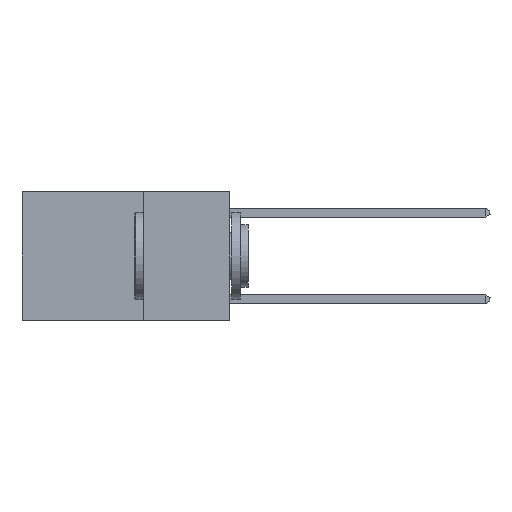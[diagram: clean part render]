
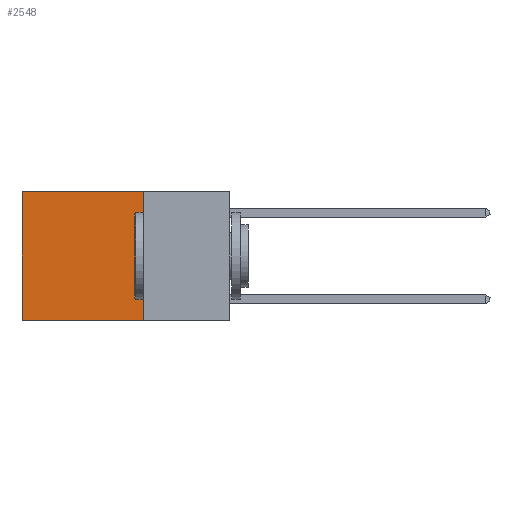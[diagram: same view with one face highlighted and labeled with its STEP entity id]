
A CAD part, left-side view. The second image highlights one B-rep face of the part: STEP entity #2548.
In plain terms, the highlighted planar face has unit normal (-1, 0, 0).
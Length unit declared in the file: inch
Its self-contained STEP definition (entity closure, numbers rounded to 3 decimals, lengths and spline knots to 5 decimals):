
#1246 = LINE ( 'NONE', #11704, #24470 ) ;
#1625 = FACE_OUTER_BOUND ( 'NONE', #7494, .T. ) ;
#2342 = CARTESIAN_POINT ( 'NONE',  ( 0.2625, 0.6, 0. ) ) ;
#2548 = ADVANCED_FACE ( 'NONE', ( #1625 ), #23971, .F. ) ;
#2975 = VERTEX_POINT ( 'NONE', #23609 ) ;
#3183 = VERTEX_POINT ( 'NONE', #4037 ) ;
#3497 = DIRECTION ( 'NONE',  ( 0., 0., -1. ) ) ;
#3573 = VECTOR ( 'NONE', #12818, 39.37008 ) ;
#4037 = CARTESIAN_POINT ( 'NONE',  ( 0.2625, 0.6, -0.37 ) ) ;
#5494 = CARTESIAN_POINT ( 'NONE',  ( 0.2625, 0.25, 0. ) ) ;
#5619 = CARTESIAN_POINT ( 'NONE',  ( 0.2625, 0.25, 0. ) ) ;
#5970 = EDGE_CURVE ( 'NONE', #22294, #3183, #23119, .T. ) ;
#7494 = EDGE_LOOP ( 'NONE', ( #20747, #15572, #9343, #20399 ) ) ;
#8528 = EDGE_CURVE ( 'NONE', #20217, #3183, #1246, .T. ) ;
#8768 = LINE ( 'NONE', #21359, #3573 ) ;
#8791 = VECTOR ( 'NONE', #21560, 39.37008 ) ;
#9343 = ORIENTED_EDGE ( 'NONE', *, *, #22044, .F. ) ;
#11704 = CARTESIAN_POINT ( 'NONE',  ( 0.2625, 0.6, 0. ) ) ;
#12243 = EDGE_CURVE ( 'NONE', #2975, #20217, #8768, .T. ) ;
#12818 = DIRECTION ( 'NONE',  ( 0., 1., 0. ) ) ;
#13393 = LINE ( 'NONE', #5619, #8791 ) ;
#15572 = ORIENTED_EDGE ( 'NONE', *, *, #5970, .F. ) ;
#17355 = CARTESIAN_POINT ( 'NONE',  ( 0.2625, 0.25, -0.37 ) ) ;
#19055 = AXIS2_PLACEMENT_3D ( 'NONE', #5494, #24105, #3497 ) ;
#19113 = DIRECTION ( 'NONE',  ( 0., 1., 0. ) ) ;
#19296 = CARTESIAN_POINT ( 'NONE',  ( 0.2625, 0.25, -0.37 ) ) ;
#20217 = VERTEX_POINT ( 'NONE', #2342 ) ;
#20399 = ORIENTED_EDGE ( 'NONE', *, *, #12243, .T. ) ;
#20747 = ORIENTED_EDGE ( 'NONE', *, *, #8528, .T. ) ;
#21359 = CARTESIAN_POINT ( 'NONE',  ( 0.2625, 0.25, 0. ) ) ;
#21560 = DIRECTION ( 'NONE',  ( 0., 0., -1. ) ) ;
#22044 = EDGE_CURVE ( 'NONE', #2975, #22294, #13393, .T. ) ;
#22294 = VERTEX_POINT ( 'NONE', #19296 ) ;
#23119 = LINE ( 'NONE', #17355, #25457 ) ;
#23609 = CARTESIAN_POINT ( 'NONE',  ( 0.2625, 0.25, 0. ) ) ;
#23971 = PLANE ( 'NONE',  #19055 ) ;
#24105 = DIRECTION ( 'NONE',  ( 1., 0., 0. ) ) ;
#24149 = DIRECTION ( 'NONE',  ( 0., 0., -1. ) ) ;
#24470 = VECTOR ( 'NONE', #24149, 39.37008 ) ;
#25457 = VECTOR ( 'NONE', #19113, 39.37008 ) ;
